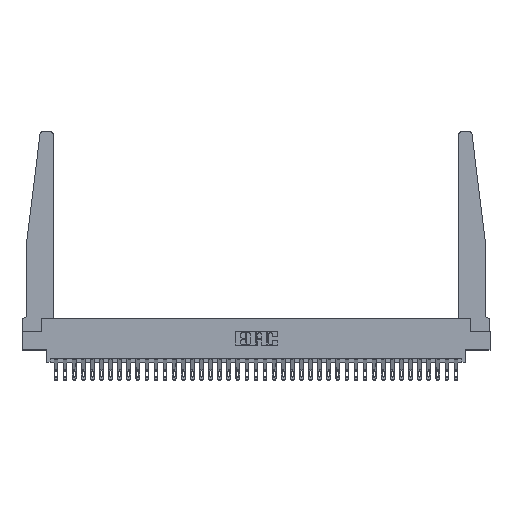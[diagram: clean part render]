
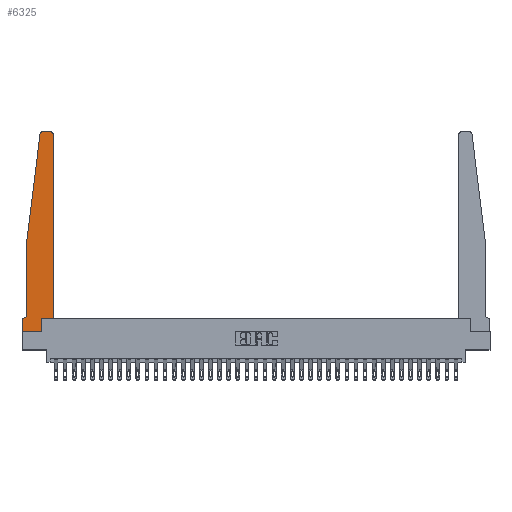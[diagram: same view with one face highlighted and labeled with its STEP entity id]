
A CAD part, top view. The second image highlights one B-rep face of the part: STEP entity #6325.
In plain terms, the highlighted planar face has unit normal (0, 0, 1).
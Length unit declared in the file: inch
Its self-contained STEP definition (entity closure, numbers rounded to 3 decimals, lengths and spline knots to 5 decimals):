
#85 = CARTESIAN_POINT ( 'NONE',  ( 0.27653, 2.72, 0.37 ) ) ;
#432 = EDGE_CURVE ( 'NONE', #2697, #33023, #23502, .T. ) ;
#483 = CARTESIAN_POINT ( 'NONE',  ( 0.065, 1.25, 0.37 ) ) ;
#514 = LINE ( 'NONE', #24369, #13748 ) ;
#872 = ORIENTED_EDGE ( 'NONE', *, *, #17698, .T. ) ;
#984 = ORIENTED_EDGE ( 'NONE', *, *, #17395, .T. ) ;
#1155 = AXIS2_PLACEMENT_3D ( 'NONE', #85, #18618, #2733 ) ;
#1215 = CARTESIAN_POINT ( 'NONE',  ( 0., 0.1875, 0.37 ) ) ;
#1223 = EDGE_LOOP ( 'NONE', ( #872, #27320, #30560, #7273, #21709, #16535, #22801, #984, #27437, #29352, #17313, #24118 ) ) ;
#1480 = CARTESIAN_POINT ( 'NONE',  ( 0.065, 0.1875, 0.37 ) ) ;
#1566 = VECTOR ( 'NONE', #33156, 39.37008 ) ;
#1682 = CARTESIAN_POINT ( 'NONE',  ( 0., 0.1875, 0.37 ) ) ;
#2015 = VECTOR ( 'NONE', #25740, 39.37008 ) ;
#2690 = VECTOR ( 'NONE', #19911, 39.37008 ) ;
#2697 = VERTEX_POINT ( 'NONE', #483 ) ;
#2733 = DIRECTION ( 'NONE',  ( 1., 0., 0. ) ) ;
#3055 = CARTESIAN_POINT ( 'NONE',  ( 0.395, 2.72, 0.37 ) ) ;
#3090 = AXIS2_PLACEMENT_3D ( 'NONE', #29848, #14039, #32516 ) ;
#3514 = LINE ( 'NONE', #17274, #2690 ) ;
#3677 = VERTEX_POINT ( 'NONE', #23306 ) ;
#3795 = FACE_OUTER_BOUND ( 'NONE', #1223, .T. ) ;
#3869 = DIRECTION ( 'NONE',  ( 0., 1., 0. ) ) ;
#4081 = VECTOR ( 'NONE', #16198, 39.37008 ) ;
#4113 = DIRECTION ( 'NONE',  ( -1., 0., 0. ) ) ;
#4319 = DIRECTION ( 'NONE',  ( 1., 0., 0. ) ) ;
#4883 = AXIS2_PLACEMENT_3D ( 'NONE', #1682, #20183, #4319 ) ;
#5718 = DIRECTION ( 'NONE',  ( 1., 0., 0. ) ) ;
#6325 = ADVANCED_FACE ( 'NONE', ( #3795 ), #17546, .T. ) ;
#7066 = CARTESIAN_POINT ( 'NONE',  ( 0.2605, 0.18, 0.37 ) ) ;
#7243 = CARTESIAN_POINT ( 'NONE',  ( 0.25, 2.75, 0.37 ) ) ;
#7273 = ORIENTED_EDGE ( 'NONE', *, *, #432, .T. ) ;
#7276 = LINE ( 'NONE', #18445, #20506 ) ;
#7962 = CARTESIAN_POINT ( 'NONE',  ( 0.425, 0.18, 0.37 ) ) ;
#8185 = CARTESIAN_POINT ( 'NONE',  ( 0.2605, 0., 0.37 ) ) ;
#8312 = VERTEX_POINT ( 'NONE', #10276 ) ;
#8724 = DIRECTION ( 'NONE',  ( 0., 1., 0. ) ) ;
#9328 = CARTESIAN_POINT ( 'NONE',  ( 0.425, 2.72, 0.37 ) ) ;
#9333 = CARTESIAN_POINT ( 'NONE',  ( 0.27653, 2.75, 0.37 ) ) ;
#10276 = CARTESIAN_POINT ( 'NONE',  ( 0., 0., 0.37 ) ) ;
#11181 = LINE ( 'NONE', #16080, #4081 ) ;
#12726 = CIRCLE ( 'NONE', #21202, 0.03 ) ;
#12872 = CIRCLE ( 'NONE', #1155, 0.03 ) ;
#13411 = LINE ( 'NONE', #1480, #33648 ) ;
#13748 = VECTOR ( 'NONE', #27004, 39.37008 ) ;
#13802 = LINE ( 'NONE', #27194, #27023 ) ;
#14039 = DIRECTION ( 'NONE',  ( 0., 0., -1. ) ) ;
#14904 = EDGE_CURVE ( 'NONE', #16126, #30700, #13802, .T. ) ;
#16080 = CARTESIAN_POINT ( 'NONE',  ( 0., 0., 0.37 ) ) ;
#16126 = VERTEX_POINT ( 'NONE', #8185 ) ;
#16198 = DIRECTION ( 'NONE',  ( 1., 0., 0. ) ) ;
#16535 = ORIENTED_EDGE ( 'NONE', *, *, #21774, .T. ) ;
#16928 = LINE ( 'NONE', #7243, #2015 ) ;
#17093 = CARTESIAN_POINT ( 'NONE',  ( 0.425, 0.18, 0.37 ) ) ;
#17274 = CARTESIAN_POINT ( 'NONE',  ( 0.065, 1.25, 0.37 ) ) ;
#17313 = ORIENTED_EDGE ( 'NONE', *, *, #19270, .T. ) ;
#17395 = EDGE_CURVE ( 'NONE', #8312, #16126, #11181, .T. ) ;
#17404 = CIRCLE ( 'NONE', #3090, 0.05 ) ;
#17546 = PLANE ( 'NONE',  #4883 ) ;
#17698 = EDGE_CURVE ( 'NONE', #23080, #33431, #16928, .T. ) ;
#17902 = CARTESIAN_POINT ( 'NONE',  ( 0.065, 0.2375, 0.37 ) ) ;
#18065 = EDGE_CURVE ( 'NONE', #33023, #3677, #17404, .T. ) ;
#18445 = CARTESIAN_POINT ( 'NONE',  ( 0., 0., 0.37 ) ) ;
#18618 = DIRECTION ( 'NONE',  ( 0., 0., 1. ) ) ;
#19270 = EDGE_CURVE ( 'NONE', #25864, #29142, #23083, .T. ) ;
#19911 = DIRECTION ( 'NONE',  ( -0.122, -0.992, 0. ) ) ;
#19989 = CARTESIAN_POINT ( 'NONE',  ( 0.065, 1.25, 0.37 ) ) ;
#20183 = DIRECTION ( 'NONE',  ( 0., 0., 1. ) ) ;
#20506 = VECTOR ( 'NONE', #31691, 39.37008 ) ;
#20812 = EDGE_CURVE ( 'NONE', #29107, #8312, #7276, .T. ) ;
#21202 = AXIS2_PLACEMENT_3D ( 'NONE', #3055, #21557, #5718 ) ;
#21557 = DIRECTION ( 'NONE',  ( 0., 0., 1. ) ) ;
#21709 = ORIENTED_EDGE ( 'NONE', *, *, #18065, .T. ) ;
#21774 = EDGE_CURVE ( 'NONE', #3677, #29107, #13411, .T. ) ;
#22239 = VECTOR ( 'NONE', #3869, 39.37008 ) ;
#22801 = ORIENTED_EDGE ( 'NONE', *, *, #20812, .T. ) ;
#23080 = VERTEX_POINT ( 'NONE', #28092 ) ;
#23083 = LINE ( 'NONE', #17093, #22239 ) ;
#23306 = CARTESIAN_POINT ( 'NONE',  ( 0.015, 0.1875, 0.37 ) ) ;
#23502 = LINE ( 'NONE', #19989, #1566 ) ;
#23553 = VERTEX_POINT ( 'NONE', #24641 ) ;
#23975 = EDGE_CURVE ( 'NONE', #33431, #23553, #12872, .T. ) ;
#24118 = ORIENTED_EDGE ( 'NONE', *, *, #29804, .T. ) ;
#24369 = CARTESIAN_POINT ( 'NONE',  ( 0.425, 0.18, 0.37 ) ) ;
#24641 = CARTESIAN_POINT ( 'NONE',  ( 0.24675, 2.72367, 0.37 ) ) ;
#25740 = DIRECTION ( 'NONE',  ( -1., 0., 0. ) ) ;
#25864 = VERTEX_POINT ( 'NONE', #7962 ) ;
#26003 = EDGE_CURVE ( 'NONE', #30700, #25864, #514, .T. ) ;
#27004 = DIRECTION ( 'NONE',  ( 1., 0., 0. ) ) ;
#27023 = VECTOR ( 'NONE', #8724, 39.37008 ) ;
#27194 = CARTESIAN_POINT ( 'NONE',  ( 0.2605, 0.18, 0.37 ) ) ;
#27320 = ORIENTED_EDGE ( 'NONE', *, *, #23975, .T. ) ;
#27437 = ORIENTED_EDGE ( 'NONE', *, *, #14904, .T. ) ;
#28092 = CARTESIAN_POINT ( 'NONE',  ( 0.395, 2.75, 0.37 ) ) ;
#29107 = VERTEX_POINT ( 'NONE', #1215 ) ;
#29142 = VERTEX_POINT ( 'NONE', #9328 ) ;
#29352 = ORIENTED_EDGE ( 'NONE', *, *, #26003, .T. ) ;
#29804 = EDGE_CURVE ( 'NONE', #29142, #23080, #12726, .T. ) ;
#29848 = CARTESIAN_POINT ( 'NONE',  ( 0.015, 0.2375, 0.37 ) ) ;
#30560 = ORIENTED_EDGE ( 'NONE', *, *, #30623, .T. ) ;
#30623 = EDGE_CURVE ( 'NONE', #23553, #2697, #3514, .T. ) ;
#30700 = VERTEX_POINT ( 'NONE', #7066 ) ;
#31691 = DIRECTION ( 'NONE',  ( 0., -1., 0. ) ) ;
#32516 = DIRECTION ( 'NONE',  ( -1., 0., 0. ) ) ;
#33023 = VERTEX_POINT ( 'NONE', #17902 ) ;
#33156 = DIRECTION ( 'NONE',  ( 0., -1., 0. ) ) ;
#33431 = VERTEX_POINT ( 'NONE', #9333 ) ;
#33648 = VECTOR ( 'NONE', #4113, 39.37008 ) ;
